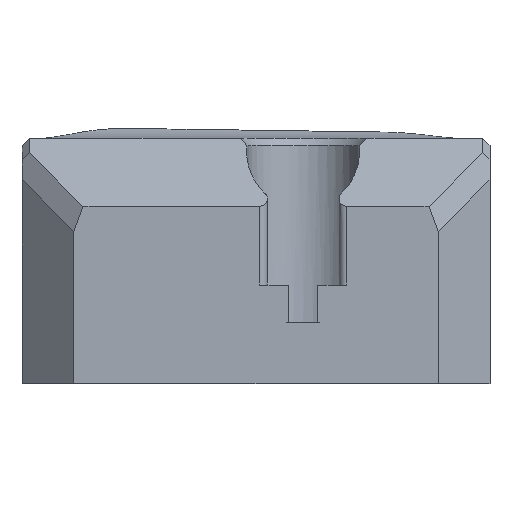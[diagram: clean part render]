
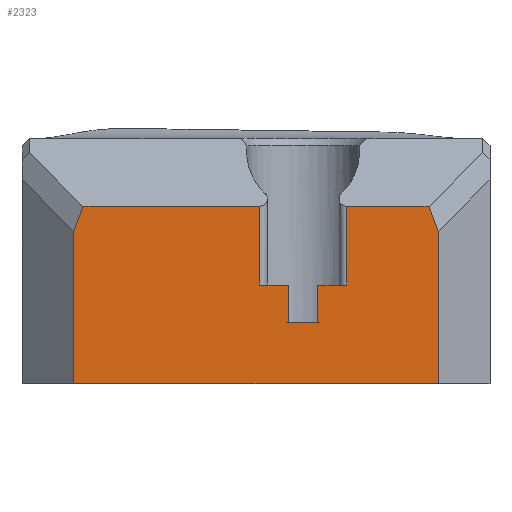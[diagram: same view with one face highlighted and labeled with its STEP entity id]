
A CAD part, front view. The second image highlights one B-rep face of the part: STEP entity #2323.
In plain terms, the highlighted planar face has unit normal (0, -1, 0).
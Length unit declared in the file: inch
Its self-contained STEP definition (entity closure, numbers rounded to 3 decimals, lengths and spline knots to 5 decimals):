
#59 = CARTESIAN_POINT ( 'NONE',  ( 2.65, -1.4, 0.51882 ) ) ;
#88 = EDGE_CURVE ( 'NONE', #2042, #2214, #1175, .T. ) ;
#91 = VERTEX_POINT ( 'NONE', #2655 ) ;
#113 = CARTESIAN_POINT ( 'NONE',  ( 1.43463, -1.4, 0.56818 ) ) ;
#124 = CARTESIAN_POINT ( 'NONE',  ( 2.33343, -1.4, 0.51882 ) ) ;
#126 = AXIS2_PLACEMENT_3D ( 'NONE', #2371, #2001, #760 ) ;
#145 = CARTESIAN_POINT ( 'NONE',  ( 2.35793, -1.4, 0.04882 ) ) ;
#186 = VERTEX_POINT ( 'NONE', #1996 ) ;
#223 = VECTOR ( 'NONE', #1637, 39.37008 ) ;
#232 = LINE ( 'NONE', #59, #333 ) ;
#239 = ORIENTED_EDGE ( 'NONE', *, *, #1449, .T. ) ;
#242 = CARTESIAN_POINT ( 'NONE',  ( 1.39207, -1.4, 1.07882 ) ) ;
#275 = LINE ( 'NONE', #703, #1681 ) ;
#298 = ORIENTED_EDGE ( 'NONE', *, *, #1080, .T. ) ;
#308 = CARTESIAN_POINT ( 'NONE',  ( 2.11522, -1.4, 0.51882 ) ) ;
#333 = VECTOR ( 'NONE', #1313, 39.37008 ) ;
#401 = VERTEX_POINT ( 'NONE', #938 ) ;
#471 = CARTESIAN_POINT ( 'NONE',  ( 1.39207, -1.4, 0.04882 ) ) ;
#477 = ORIENTED_EDGE ( 'NONE', *, *, #2460, .T. ) ;
#523 = CARTESIAN_POINT ( 'NONE',  ( 2.03841, -1.4, 0.31 ) ) ;
#536 = EDGE_CURVE ( 'NONE', #401, #2299, #1777, .T. ) ;
#588 = ORIENTED_EDGE ( 'NONE', *, *, #536, .T. ) ;
#647 = LINE ( 'NONE', #2502, #860 ) ;
#685 = EDGE_CURVE ( 'NONE', #2027, #2265, #232, .T. ) ;
#687 = EDGE_CURVE ( 'NONE', #927, #2532, #2332, .T. ) ;
#703 = CARTESIAN_POINT ( 'NONE',  ( 1.96159, -1.4, 1.07882 ) ) ;
#760 = DIRECTION ( 'NONE',  ( -1., 0., 0. ) ) ;
#779 = LINE ( 'NONE', #1586, #1710 ) ;
#788 = VECTOR ( 'NONE', #2588, 39.37008 ) ;
#792 = LINE ( 'NONE', #1139, #1801 ) ;
#813 = CARTESIAN_POINT ( 'NONE',  ( 2.35793, -1.4, 1.07882 ) ) ;
#856 = DIRECTION ( 'NONE',  ( 0., 0., -1. ) ) ;
#860 = VECTOR ( 'NONE', #2676, 39.37008 ) ;
#927 = VERTEX_POINT ( 'NONE', #145 ) ;
#930 = DIRECTION ( 'NONE',  ( -1., 0., 0. ) ) ;
#938 = CARTESIAN_POINT ( 'NONE',  ( 1.88478, -1.4, 0.51882 ) ) ;
#939 = ORIENTED_EDGE ( 'NONE', *, *, #1789, .T. ) ;
#998 = DIRECTION ( 'NONE',  ( -1., 0., 0. ) ) ;
#1027 = VECTOR ( 'NONE', #2061, 39.37008 ) ;
#1063 = ORIENTED_EDGE ( 'NONE', *, *, #2218, .T. ) ;
#1080 = EDGE_CURVE ( 'NONE', #1091, #2532, #1664, .T. ) ;
#1091 = VERTEX_POINT ( 'NONE', #2514 ) ;
#1130 = ORIENTED_EDGE ( 'NONE', *, *, #2120, .F. ) ;
#1139 = CARTESIAN_POINT ( 'NONE',  ( 2.29627, -1.4, 0.62036 ) ) ;
#1148 = EDGE_CURVE ( 'NONE', #2214, #2612, #2213, .T. ) ;
#1175 = LINE ( 'NONE', #1419, #1559 ) ;
#1237 = ORIENTED_EDGE ( 'NONE', *, *, #685, .T. ) ;
#1299 = DIRECTION ( 'NONE',  ( -1., 0., 0. ) ) ;
#1301 = EDGE_CURVE ( 'NONE', #91, #401, #647, .T. ) ;
#1313 = DIRECTION ( 'NONE',  ( -1., 0., 0. ) ) ;
#1343 = CARTESIAN_POINT ( 'NONE',  ( 2.03841, -1.4, 1.07882 ) ) ;
#1400 = EDGE_CURVE ( 'NONE', #2265, #2042, #1632, .T. ) ;
#1419 = CARTESIAN_POINT ( 'NONE',  ( 3.52262, -1.4, 0.31 ) ) ;
#1437 = VECTOR ( 'NONE', #2032, 39.37008 ) ;
#1449 = EDGE_CURVE ( 'NONE', #2612, #186, #779, .T. ) ;
#1464 = EDGE_CURVE ( 'NONE', #2067, #2027, #792, .T. ) ;
#1469 = CARTESIAN_POINT ( 'NONE',  ( 1.25, -1.4, 0.04882 ) ) ;
#1526 = DIRECTION ( 'NONE',  ( 0., 0., 1. ) ) ;
#1559 = VECTOR ( 'NONE', #998, 39.37008 ) ;
#1568 = FACE_OUTER_BOUND ( 'NONE', #1757, .T. ) ;
#1586 = CARTESIAN_POINT ( 'NONE',  ( 2., -1.4, 0.21 ) ) ;
#1587 = DIRECTION ( 'NONE',  ( 0., 0., -1. ) ) ;
#1627 = CARTESIAN_POINT ( 'NONE',  ( 1.96159, -1.4, 0.31 ) ) ;
#1632 = LINE ( 'NONE', #2461, #1027 ) ;
#1637 = DIRECTION ( 'NONE',  ( 0., 0., -1. ) ) ;
#1664 = LINE ( 'NONE', #242, #2244 ) ;
#1681 = VECTOR ( 'NONE', #1526, 39.37008 ) ;
#1710 = VECTOR ( 'NONE', #2434, 39.37008 ) ;
#1749 = PLANE ( 'NONE',  #126 ) ;
#1757 = EDGE_LOOP ( 'NONE', ( #588, #1063, #298, #2510, #1130, #2639, #1237, #1984, #1878, #2193, #239, #939, #477, #2288 ) ) ;
#1777 = LINE ( 'NONE', #1967, #2003 ) ;
#1782 = LINE ( 'NONE', #113, #788 ) ;
#1789 = EDGE_CURVE ( 'NONE', #186, #2431, #275, .T. ) ;
#1801 = VECTOR ( 'NONE', #2167, 39.37008 ) ;
#1854 = CARTESIAN_POINT ( 'NONE',  ( 2.11522, -1.4, 0.31 ) ) ;
#1867 = LINE ( 'NONE', #813, #223 ) ;
#1878 = ORIENTED_EDGE ( 'NONE', *, *, #88, .T. ) ;
#1967 = CARTESIAN_POINT ( 'NONE',  ( 2.65, -1.4, 0.51882 ) ) ;
#1984 = ORIENTED_EDGE ( 'NONE', *, *, #1400, .T. ) ;
#1996 = CARTESIAN_POINT ( 'NONE',  ( 1.96159, -1.4, 0.21 ) ) ;
#2001 = DIRECTION ( 'NONE',  ( 0., 1., 0. ) ) ;
#2003 = VECTOR ( 'NONE', #930, 39.37008 ) ;
#2027 = VERTEX_POINT ( 'NONE', #124 ) ;
#2032 = DIRECTION ( 'NONE',  ( -1., 0., 0. ) ) ;
#2042 = VERTEX_POINT ( 'NONE', #1854 ) ;
#2058 = CARTESIAN_POINT ( 'NONE',  ( 3.52262, -1.4, 0.31 ) ) ;
#2061 = DIRECTION ( 'NONE',  ( 0., 0., -1. ) ) ;
#2067 = VERTEX_POINT ( 'NONE', #2290 ) ;
#2087 = LINE ( 'NONE', #2058, #1437 ) ;
#2120 = EDGE_CURVE ( 'NONE', #2067, #927, #1867, .T. ) ;
#2167 = DIRECTION ( 'NONE',  ( -0.344, 0., 0.939 ) ) ;
#2190 = CARTESIAN_POINT ( 'NONE',  ( 2.03841, -1.4, 0.21 ) ) ;
#2193 = ORIENTED_EDGE ( 'NONE', *, *, #1148, .T. ) ;
#2213 = LINE ( 'NONE', #1343, #2464 ) ;
#2214 = VERTEX_POINT ( 'NONE', #523 ) ;
#2218 = EDGE_CURVE ( 'NONE', #2299, #1091, #1782, .T. ) ;
#2244 = VECTOR ( 'NONE', #856, 39.37008 ) ;
#2265 = VERTEX_POINT ( 'NONE', #308 ) ;
#2288 = ORIENTED_EDGE ( 'NONE', *, *, #1301, .T. ) ;
#2290 = CARTESIAN_POINT ( 'NONE',  ( 2.35793, -1.4, 0.4519 ) ) ;
#2299 = VERTEX_POINT ( 'NONE', #2384 ) ;
#2323 = ADVANCED_FACE ( 'NONE', ( #1568 ), #1749, .F. ) ;
#2332 = LINE ( 'NONE', #1469, #2675 ) ;
#2371 = CARTESIAN_POINT ( 'NONE',  ( 2.65, -1.4, 0.69882 ) ) ;
#2384 = CARTESIAN_POINT ( 'NONE',  ( 1.41657, -1.4, 0.51882 ) ) ;
#2431 = VERTEX_POINT ( 'NONE', #1627 ) ;
#2434 = DIRECTION ( 'NONE',  ( -1., 0., 0. ) ) ;
#2460 = EDGE_CURVE ( 'NONE', #2431, #91, #2087, .T. ) ;
#2461 = CARTESIAN_POINT ( 'NONE',  ( 2.11522, -1.4, 0.31 ) ) ;
#2464 = VECTOR ( 'NONE', #1587, 39.37008 ) ;
#2502 = CARTESIAN_POINT ( 'NONE',  ( 1.88478, -1.4, 0.51882 ) ) ;
#2510 = ORIENTED_EDGE ( 'NONE', *, *, #687, .F. ) ;
#2514 = CARTESIAN_POINT ( 'NONE',  ( 1.39207, -1.4, 0.4519 ) ) ;
#2532 = VERTEX_POINT ( 'NONE', #471 ) ;
#2588 = DIRECTION ( 'NONE',  ( -0.344, 0., -0.939 ) ) ;
#2612 = VERTEX_POINT ( 'NONE', #2190 ) ;
#2639 = ORIENTED_EDGE ( 'NONE', *, *, #1464, .T. ) ;
#2655 = CARTESIAN_POINT ( 'NONE',  ( 1.88478, -1.4, 0.31 ) ) ;
#2675 = VECTOR ( 'NONE', #1299, 39.37008 ) ;
#2676 = DIRECTION ( 'NONE',  ( 0., 0., 1. ) ) ;
